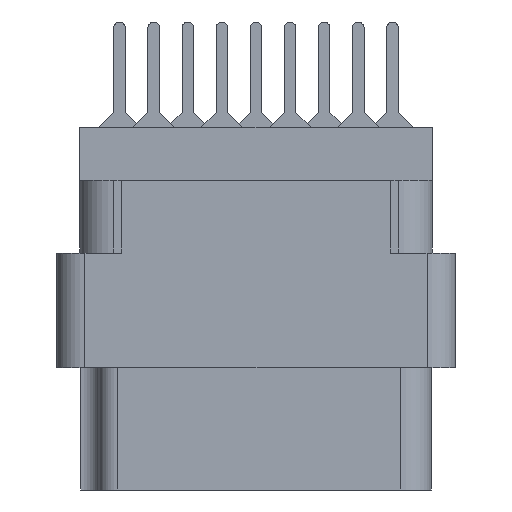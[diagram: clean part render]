
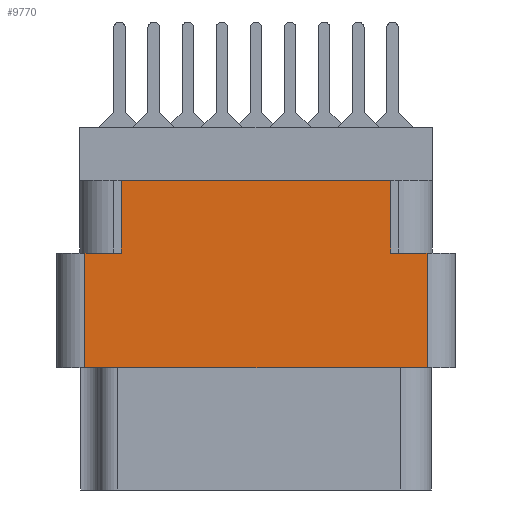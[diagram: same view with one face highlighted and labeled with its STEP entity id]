
A CAD part, left-side view. The second image highlights one B-rep face of the part: STEP entity #9770.
In plain terms, the highlighted planar face has unit normal (-1, 0, 0).
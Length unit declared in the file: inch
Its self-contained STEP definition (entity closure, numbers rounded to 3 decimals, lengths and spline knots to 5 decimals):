
#170 = EDGE_CURVE ( 'NONE', #24151, #16765, #19322, .T. ) ;
#1042 = ORIENTED_EDGE ( 'NONE', *, *, #1507, .T. ) ;
#1391 = LINE ( 'NONE', #11672, #26151 ) ;
#1507 = EDGE_CURVE ( 'NONE', #33451, #18408, #5829, .T. ) ;
#1570 = CARTESIAN_POINT ( 'NONE',  ( -1., -0.296, -0.117 ) ) ;
#1765 = LINE ( 'NONE', #16470, #13943 ) ;
#2438 = EDGE_CURVE ( 'NONE', #9818, #3536, #4906, .T. ) ;
#2472 = CARTESIAN_POINT ( 'NONE',  ( -1., -0.376, -0.277 ) ) ;
#3536 = VERTEX_POINT ( 'NONE', #2472 ) ;
#3885 = ORIENTED_EDGE ( 'NONE', *, *, #12989, .F. ) ;
#4531 = VECTOR ( 'NONE', #30532, 39.37008 ) ;
#4578 = AXIS2_PLACEMENT_3D ( 'NONE', #21324, #18400, #7877 ) ;
#4719 = LINE ( 'NONE', #16415, #8486 ) ;
#4769 = ORIENTED_EDGE ( 'NONE', *, *, #170, .F. ) ;
#4906 = LINE ( 'NONE', #29518, #23096 ) ;
#5829 = LINE ( 'NONE', #8932, #4531 ) ;
#6659 = DIRECTION ( 'NONE',  ( 0., -1., 0. ) ) ;
#7877 = DIRECTION ( 'NONE',  ( 0., 0., 1. ) ) ;
#8486 = VECTOR ( 'NONE', #24143, 39.37008 ) ;
#8551 = VERTEX_POINT ( 'NONE', #30232 ) ;
#8932 = CARTESIAN_POINT ( 'NONE',  ( -1., 0.376, -0.798 ) ) ;
#8987 = VECTOR ( 'NONE', #14340, 39.37008 ) ;
#9286 = CARTESIAN_POINT ( 'NONE',  ( -1., 0.296, -0.277 ) ) ;
#9683 = DIRECTION ( 'NONE',  ( 0., -1., 0. ) ) ;
#9770 = ADVANCED_FACE ( 'NONE', ( #31367 ), #26266, .T. ) ;
#9818 = VERTEX_POINT ( 'NONE', #15828 ) ;
#9892 = ORIENTED_EDGE ( 'NONE', *, *, #28936, .T. ) ;
#10538 = ORIENTED_EDGE ( 'NONE', *, *, #2438, .T. ) ;
#11672 = CARTESIAN_POINT ( 'NONE',  ( -1., -0.296, -0.277 ) ) ;
#12989 = EDGE_CURVE ( 'NONE', #9818, #18408, #4719, .T. ) ;
#13939 = LINE ( 'NONE', #22807, #25666 ) ;
#13943 = VECTOR ( 'NONE', #27119, 39.37008 ) ;
#14340 = DIRECTION ( 'NONE',  ( 0., 0., 1. ) ) ;
#14819 = CARTESIAN_POINT ( 'NONE',  ( -1., 0.376, -0.277 ) ) ;
#15828 = CARTESIAN_POINT ( 'NONE',  ( -1., -0.376, -0.529 ) ) ;
#16415 = CARTESIAN_POINT ( 'NONE',  ( -1., 0., -0.529 ) ) ;
#16470 = CARTESIAN_POINT ( 'NONE',  ( -1., 0., -0.277 ) ) ;
#16765 = VERTEX_POINT ( 'NONE', #1570 ) ;
#17651 = VECTOR ( 'NONE', #6659, 39.37008 ) ;
#18400 = DIRECTION ( 'NONE',  ( -1., 0., 0. ) ) ;
#18408 = VERTEX_POINT ( 'NONE', #19196 ) ;
#19196 = CARTESIAN_POINT ( 'NONE',  ( -1., 0.376, -0.529 ) ) ;
#19322 = LINE ( 'NONE', #25276, #17651 ) ;
#19723 = EDGE_CURVE ( 'NONE', #8551, #24151, #23248, .T. ) ;
#21063 = DIRECTION ( 'NONE',  ( 0., 0., 1. ) ) ;
#21324 = CARTESIAN_POINT ( 'NONE',  ( -1., -0.438, -0.798 ) ) ;
#22807 = CARTESIAN_POINT ( 'NONE',  ( -1., 0., -0.277 ) ) ;
#23096 = VECTOR ( 'NONE', #21063, 39.37008 ) ;
#23248 = LINE ( 'NONE', #9286, #8987 ) ;
#24055 = EDGE_LOOP ( 'NONE', ( #24809, #1042, #3885, #10538, #26136, #9892, #4769, #33803 ) ) ;
#24143 = DIRECTION ( 'NONE',  ( 0., 1., 0. ) ) ;
#24151 = VERTEX_POINT ( 'NONE', #31702 ) ;
#24809 = ORIENTED_EDGE ( 'NONE', *, *, #27243, .F. ) ;
#25276 = CARTESIAN_POINT ( 'NONE',  ( -1., 0.438, -0.117 ) ) ;
#25666 = VECTOR ( 'NONE', #9683, 39.37008 ) ;
#26136 = ORIENTED_EDGE ( 'NONE', *, *, #29461, .F. ) ;
#26151 = VECTOR ( 'NONE', #34177, 39.37008 ) ;
#26266 = PLANE ( 'NONE',  #4578 ) ;
#27119 = DIRECTION ( 'NONE',  ( 0., -1., 0. ) ) ;
#27243 = EDGE_CURVE ( 'NONE', #33451, #8551, #13939, .T. ) ;
#28936 = EDGE_CURVE ( 'NONE', #28972, #16765, #1391, .T. ) ;
#28972 = VERTEX_POINT ( 'NONE', #33419 ) ;
#29461 = EDGE_CURVE ( 'NONE', #28972, #3536, #1765, .T. ) ;
#29518 = CARTESIAN_POINT ( 'NONE',  ( -1., -0.376, -0.798 ) ) ;
#30232 = CARTESIAN_POINT ( 'NONE',  ( -1., 0.296, -0.277 ) ) ;
#30532 = DIRECTION ( 'NONE',  ( 0., 0., -1. ) ) ;
#31367 = FACE_OUTER_BOUND ( 'NONE', #24055, .T. ) ;
#31702 = CARTESIAN_POINT ( 'NONE',  ( -1., 0.296, -0.117 ) ) ;
#33419 = CARTESIAN_POINT ( 'NONE',  ( -1., -0.296, -0.277 ) ) ;
#33451 = VERTEX_POINT ( 'NONE', #14819 ) ;
#33803 = ORIENTED_EDGE ( 'NONE', *, *, #19723, .F. ) ;
#34177 = DIRECTION ( 'NONE',  ( 0., 0., 1. ) ) ;
